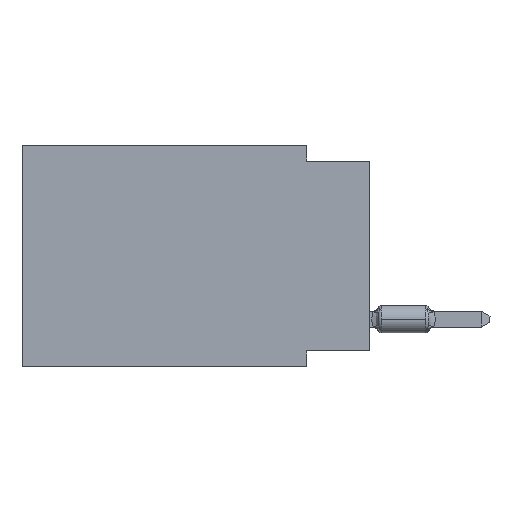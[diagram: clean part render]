
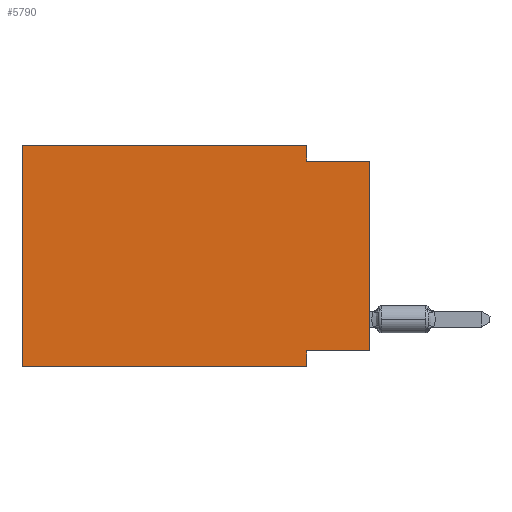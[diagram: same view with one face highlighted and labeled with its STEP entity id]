
A CAD part, left-side view. The second image highlights one B-rep face of the part: STEP entity #5790.
In plain terms, the highlighted planar face has unit normal (-1, 0, 0).
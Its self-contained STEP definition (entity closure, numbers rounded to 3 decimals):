
#54 = ORIENTED_EDGE ( 'NONE', *, *, #6360, .F. ) ;
#63 = AXIS2_PLACEMENT_3D ( 'NONE', #208, #142, #2282 ) ;
#142 = DIRECTION ( 'NONE',  ( 1., 0., 0. ) ) ;
#208 = CARTESIAN_POINT ( 'NONE',  ( 0., 13.97, 0. ) ) ;
#351 = VERTEX_POINT ( 'NONE', #12216 ) ;
#389 = CARTESIAN_POINT ( 'NONE',  ( 0., 0., -8.255 ) ) ;
#595 = CARTESIAN_POINT ( 'NONE',  ( 0., 2.54, -8.89 ) ) ;
#699 = LINE ( 'NONE', #12749, #7237 ) ;
#843 = CARTESIAN_POINT ( 'NONE',  ( 0., 13.97, -8.89 ) ) ;
#1120 = CARTESIAN_POINT ( 'NONE',  ( 0., 13.97, 0. ) ) ;
#1138 = FACE_OUTER_BOUND ( 'NONE', #1454, .T. ) ;
#1454 = EDGE_LOOP ( 'NONE', ( #7091, #54, #11455, #11220, #10128, #8178, #9936, #6331 ) ) ;
#1747 = CARTESIAN_POINT ( 'NONE',  ( 0., 13.97, 0. ) ) ;
#1763 = DIRECTION ( 'NONE',  ( 0., 0., 1. ) ) ;
#2262 = VECTOR ( 'NONE', #7835, 1000. ) ;
#2282 = DIRECTION ( 'NONE',  ( 0., 0., -1. ) ) ;
#3143 = EDGE_CURVE ( 'NONE', #8692, #7008, #9895, .T. ) ;
#3363 = PLANE ( 'NONE',  #63 ) ;
#3524 = CARTESIAN_POINT ( 'NONE',  ( 0., 2.54, 0. ) ) ;
#3708 = CARTESIAN_POINT ( 'NONE',  ( 0., 2.54, 0. ) ) ;
#3731 = CARTESIAN_POINT ( 'NONE',  ( 0., 0., -0.635 ) ) ;
#4156 = VECTOR ( 'NONE', #13151, 1000. ) ;
#4348 = EDGE_CURVE ( 'NONE', #9260, #8692, #10651, .T. ) ;
#4414 = VERTEX_POINT ( 'NONE', #10280 ) ;
#4714 = DIRECTION ( 'NONE',  ( 0., 0., -1. ) ) ;
#5163 = EDGE_CURVE ( 'NONE', #12205, #5896, #699, .T. ) ;
#5790 = ADVANCED_FACE ( 'NONE', ( #1138 ), #3363, .F. ) ;
#5896 = VERTEX_POINT ( 'NONE', #6313 ) ;
#6313 = CARTESIAN_POINT ( 'NONE',  ( 0., 2.54, -8.255 ) ) ;
#6331 = ORIENTED_EDGE ( 'NONE', *, *, #5163, .F. ) ;
#6360 = EDGE_CURVE ( 'NONE', #7008, #4414, #10555, .T. ) ;
#6379 = VECTOR ( 'NONE', #6735, 1000. ) ;
#6735 = DIRECTION ( 'NONE',  ( 0., -1., 0. ) ) ;
#7008 = VERTEX_POINT ( 'NONE', #10106 ) ;
#7091 = ORIENTED_EDGE ( 'NONE', *, *, #7651, .T. ) ;
#7237 = VECTOR ( 'NONE', #9725, 1000. ) ;
#7642 = VECTOR ( 'NONE', #11418, 1000. ) ;
#7651 = EDGE_CURVE ( 'NONE', #12205, #4414, #8776, .T. ) ;
#7833 = VECTOR ( 'NONE', #4714, 1000. ) ;
#7835 = DIRECTION ( 'NONE',  ( 0., -1., 0. ) ) ;
#7971 = EDGE_CURVE ( 'NONE', #5896, #9365, #9938, .T. ) ;
#8178 = ORIENTED_EDGE ( 'NONE', *, *, #8415, .T. ) ;
#8415 = EDGE_CURVE ( 'NONE', #351, #9365, #8855, .T. ) ;
#8692 = VERTEX_POINT ( 'NONE', #3524 ) ;
#8776 = LINE ( 'NONE', #12873, #9786 ) ;
#8855 = LINE ( 'NONE', #843, #4156 ) ;
#9102 = VECTOR ( 'NONE', #12902, 1000. ) ;
#9260 = VERTEX_POINT ( 'NONE', #1747 ) ;
#9365 = VERTEX_POINT ( 'NONE', #11038 ) ;
#9725 = DIRECTION ( 'NONE',  ( 0., 1., 0. ) ) ;
#9786 = VECTOR ( 'NONE', #1763, 1000. ) ;
#9895 = LINE ( 'NONE', #3708, #7833 ) ;
#9936 = ORIENTED_EDGE ( 'NONE', *, *, #7971, .F. ) ;
#9938 = LINE ( 'NONE', #595, #9102 ) ;
#10106 = CARTESIAN_POINT ( 'NONE',  ( 0., 2.54, -0.635 ) ) ;
#10128 = ORIENTED_EDGE ( 'NONE', *, *, #12013, .F. ) ;
#10280 = CARTESIAN_POINT ( 'NONE',  ( 0., 0., -0.635 ) ) ;
#10555 = LINE ( 'NONE', #3731, #2262 ) ;
#10651 = LINE ( 'NONE', #10851, #6379 ) ;
#10851 = CARTESIAN_POINT ( 'NONE',  ( 0., 13.97, 0. ) ) ;
#11038 = CARTESIAN_POINT ( 'NONE',  ( 0., 2.54, -8.89 ) ) ;
#11220 = ORIENTED_EDGE ( 'NONE', *, *, #4348, .F. ) ;
#11418 = DIRECTION ( 'NONE',  ( 0., 0., 1. ) ) ;
#11455 = ORIENTED_EDGE ( 'NONE', *, *, #3143, .F. ) ;
#11484 = LINE ( 'NONE', #1120, #7642 ) ;
#12013 = EDGE_CURVE ( 'NONE', #351, #9260, #11484, .T. ) ;
#12205 = VERTEX_POINT ( 'NONE', #389 ) ;
#12216 = CARTESIAN_POINT ( 'NONE',  ( 0., 13.97, -8.89 ) ) ;
#12749 = CARTESIAN_POINT ( 'NONE',  ( 0., 0., -8.255 ) ) ;
#12873 = CARTESIAN_POINT ( 'NONE',  ( 0., 0., 0. ) ) ;
#12902 = DIRECTION ( 'NONE',  ( 0., 0., -1. ) ) ;
#13151 = DIRECTION ( 'NONE',  ( 0., -1., 0. ) ) ;
